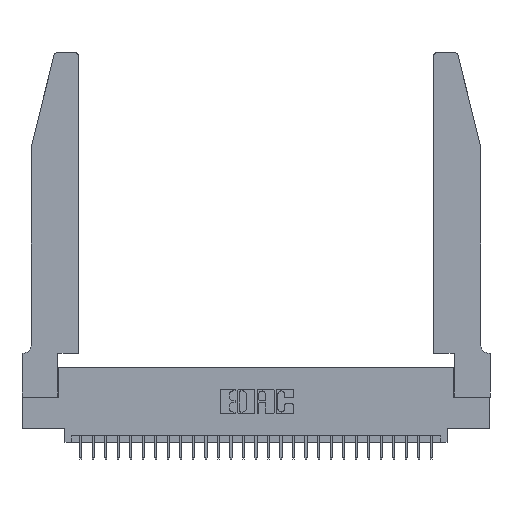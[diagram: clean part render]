
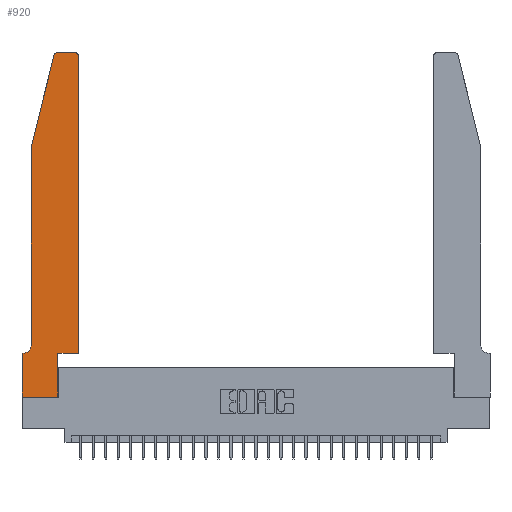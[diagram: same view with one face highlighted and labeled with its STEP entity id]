
A CAD part, top view. The second image highlights one B-rep face of the part: STEP entity #920.
In plain terms, the highlighted planar face has unit normal (0, 0, 1).
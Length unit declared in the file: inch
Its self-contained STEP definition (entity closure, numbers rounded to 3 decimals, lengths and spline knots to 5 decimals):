
#200 = PLANE ( 'NONE',  #16085 ) ;
#347 = LINE ( 'NONE', #27512, #17475 ) ;
#394 = EDGE_CURVE ( 'NONE', #6645, #23849, #20390, .T. ) ;
#507 = FACE_OUTER_BOUND ( 'NONE', #16036, .T. ) ;
#920 = ADVANCED_FACE ( 'NONE', ( #507 ), #200, .T. ) ;
#1801 = CARTESIAN_POINT ( 'NONE',  ( 0.0755, 0.35, 0.37 ) ) ;
#1813 = CARTESIAN_POINT ( 'NONE',  ( 0.0755, 2., 0.37 ) ) ;
#2017 = CARTESIAN_POINT ( 'NONE',  ( 0., 0., 0.37 ) ) ;
#2040 = VERTEX_POINT ( 'NONE', #2017 ) ;
#2989 = DIRECTION ( 'NONE',  ( -1., 0., 0. ) ) ;
#3089 = EDGE_CURVE ( 'NONE', #14643, #23645, #22229, .T. ) ;
#3415 = ORIENTED_EDGE ( 'NONE', *, *, #20732, .T. ) ;
#3640 = VECTOR ( 'NONE', #22770, 39.37008 ) ;
#4037 = CARTESIAN_POINT ( 'NONE',  ( 0.4505, 0.35, 0.37 ) ) ;
#4064 = LINE ( 'NONE', #24223, #6654 ) ;
#4484 = ORIENTED_EDGE ( 'NONE', *, *, #28660, .T. ) ;
#4575 = ORIENTED_EDGE ( 'NONE', *, *, #14215, .T. ) ;
#4797 = CARTESIAN_POINT ( 'NONE',  ( 0.284, 2.75, 0.37 ) ) ;
#5104 = CARTESIAN_POINT ( 'NONE',  ( 0., 0.35, 0.37 ) ) ;
#5279 = EDGE_CURVE ( 'NONE', #23849, #8082, #4064, .T. ) ;
#5374 = CARTESIAN_POINT ( 'NONE',  ( 0.2605, 2.75, 0.37 ) ) ;
#6134 = ORIENTED_EDGE ( 'NONE', *, *, #21720, .T. ) ;
#6453 = DIRECTION ( 'NONE',  ( -0.239, -0.971, 0. ) ) ;
#6645 = VERTEX_POINT ( 'NONE', #4797 ) ;
#6654 = VECTOR ( 'NONE', #6453, 39.37008 ) ;
#6843 = DIRECTION ( 'NONE',  ( 0., 1., 0. ) ) ;
#7436 = VECTOR ( 'NONE', #25301, 39.37008 ) ;
#7520 = DIRECTION ( 'NONE',  ( 0., 0., 1. ) ) ;
#7911 = AXIS2_PLACEMENT_3D ( 'NONE', #22703, #14601, #21188 ) ;
#8021 = VERTEX_POINT ( 'NONE', #9719 ) ;
#8082 = VERTEX_POINT ( 'NONE', #1813 ) ;
#8437 = LINE ( 'NONE', #26649, #12352 ) ;
#8638 = ORIENTED_EDGE ( 'NONE', *, *, #3089, .T. ) ;
#8874 = VECTOR ( 'NONE', #15815, 39.37008 ) ;
#9189 = CARTESIAN_POINT ( 'NONE',  ( 0.4505, 0.35, 0.37 ) ) ;
#9289 = ORIENTED_EDGE ( 'NONE', *, *, #21167, .T. ) ;
#9345 = DIRECTION ( 'NONE',  ( 1., 0., 0. ) ) ;
#9667 = CARTESIAN_POINT ( 'NONE',  ( 0.2865, 0., 0.37 ) ) ;
#9719 = CARTESIAN_POINT ( 'NONE',  ( 0.2865, 0.35, 0.37 ) ) ;
#10353 = VECTOR ( 'NONE', #10896, 39.37008 ) ;
#10664 = VERTEX_POINT ( 'NONE', #26096 ) ;
#10896 = DIRECTION ( 'NONE',  ( -1., 0., 0. ) ) ;
#10957 = VERTEX_POINT ( 'NONE', #18164 ) ;
#11267 = ORIENTED_EDGE ( 'NONE', *, *, #394, .T. ) ;
#11859 = CARTESIAN_POINT ( 'NONE',  ( 0., 0., 0.37 ) ) ;
#12352 = VECTOR ( 'NONE', #17390, 39.37008 ) ;
#14215 = EDGE_CURVE ( 'NONE', #10664, #6645, #25700, .T. ) ;
#14601 = DIRECTION ( 'NONE',  ( 0., 0., -1. ) ) ;
#14643 = VERTEX_POINT ( 'NONE', #21169 ) ;
#15305 = EDGE_CURVE ( 'NONE', #23645, #2040, #20818, .T. ) ;
#15375 = EDGE_CURVE ( 'NONE', #10957, #10664, #24615, .T. ) ;
#15485 = VECTOR ( 'NONE', #2989, 39.37008 ) ;
#15815 = DIRECTION ( 'NONE',  ( 1., 0., 0. ) ) ;
#16036 = EDGE_LOOP ( 'NONE', ( #4575, #11267, #16542, #6134, #18765, #8638, #23302, #3415, #18754, #9289, #4484, #24400 ) ) ;
#16085 = AXIS2_PLACEMENT_3D ( 'NONE', #5104, #18556, #27359 ) ;
#16542 = ORIENTED_EDGE ( 'NONE', *, *, #5279, .T. ) ;
#16635 = VERTEX_POINT ( 'NONE', #24690 ) ;
#17390 = DIRECTION ( 'NONE',  ( 0., 1., 0. ) ) ;
#17475 = VECTOR ( 'NONE', #25126, 39.37008 ) ;
#18074 = CARTESIAN_POINT ( 'NONE',  ( 0., 0., 0.37 ) ) ;
#18164 = CARTESIAN_POINT ( 'NONE',  ( 0.4505, 2.72, 0.37 ) ) ;
#18208 = LINE ( 'NONE', #27311, #21998 ) ;
#18556 = DIRECTION ( 'NONE',  ( 0., 0., 1. ) ) ;
#18601 = EDGE_CURVE ( 'NONE', #16635, #14643, #19356, .T. ) ;
#18725 = CARTESIAN_POINT ( 'NONE',  ( 0.4205, 2.72, 0.37 ) ) ;
#18754 = ORIENTED_EDGE ( 'NONE', *, *, #26317, .T. ) ;
#18765 = ORIENTED_EDGE ( 'NONE', *, *, #18601, .T. ) ;
#18915 = VERTEX_POINT ( 'NONE', #9667 ) ;
#19356 = CIRCLE ( 'NONE', #7911, 0.07 ) ;
#20390 = CIRCLE ( 'NONE', #29455, 0.03 ) ;
#20539 = VERTEX_POINT ( 'NONE', #4037 ) ;
#20732 = EDGE_CURVE ( 'NONE', #2040, #18915, #29428, .T. ) ;
#20818 = LINE ( 'NONE', #11859, #7436 ) ;
#21120 = DIRECTION ( 'NONE',  ( 0., 0., 1. ) ) ;
#21167 = EDGE_CURVE ( 'NONE', #8021, #20539, #25458, .T. ) ;
#21169 = CARTESIAN_POINT ( 'NONE',  ( 0.0055, 0.35, 0.37 ) ) ;
#21188 = DIRECTION ( 'NONE',  ( -1., 0., 0. ) ) ;
#21720 = EDGE_CURVE ( 'NONE', #8082, #16635, #347, .T. ) ;
#21998 = VECTOR ( 'NONE', #6843, 39.37008 ) ;
#22229 = LINE ( 'NONE', #1801, #10353 ) ;
#22693 = AXIS2_PLACEMENT_3D ( 'NONE', #18725, #7520, #27832 ) ;
#22703 = CARTESIAN_POINT ( 'NONE',  ( 0.0055, 0.42, 0.37 ) ) ;
#22770 = DIRECTION ( 'NONE',  ( 1., 0., 0. ) ) ;
#23302 = ORIENTED_EDGE ( 'NONE', *, *, #15305, .T. ) ;
#23645 = VERTEX_POINT ( 'NONE', #26277 ) ;
#23849 = VERTEX_POINT ( 'NONE', #27601 ) ;
#24223 = CARTESIAN_POINT ( 'NONE',  ( 0.0755, 2., 0.37 ) ) ;
#24400 = ORIENTED_EDGE ( 'NONE', *, *, #15375, .T. ) ;
#24615 = CIRCLE ( 'NONE', #22693, 0.03 ) ;
#24690 = CARTESIAN_POINT ( 'NONE',  ( 0.0755, 0.42, 0.37 ) ) ;
#25126 = DIRECTION ( 'NONE',  ( 0., -1., 0. ) ) ;
#25301 = DIRECTION ( 'NONE',  ( 0., -1., 0. ) ) ;
#25458 = LINE ( 'NONE', #9189, #3640 ) ;
#25700 = LINE ( 'NONE', #5374, #15485 ) ;
#26096 = CARTESIAN_POINT ( 'NONE',  ( 0.4205, 2.75, 0.37 ) ) ;
#26277 = CARTESIAN_POINT ( 'NONE',  ( 0., 0.35, 0.37 ) ) ;
#26317 = EDGE_CURVE ( 'NONE', #18915, #8021, #8437, .T. ) ;
#26649 = CARTESIAN_POINT ( 'NONE',  ( 0.2865, 0.35, 0.37 ) ) ;
#27311 = CARTESIAN_POINT ( 'NONE',  ( 0.4505, 0.35, 0.37 ) ) ;
#27359 = DIRECTION ( 'NONE',  ( 1., 0., 0. ) ) ;
#27512 = CARTESIAN_POINT ( 'NONE',  ( 0.0755, 2., 0.37 ) ) ;
#27601 = CARTESIAN_POINT ( 'NONE',  ( 0.25487, 2.72718, 0.37 ) ) ;
#27832 = DIRECTION ( 'NONE',  ( 1., 0., 0. ) ) ;
#28148 = CARTESIAN_POINT ( 'NONE',  ( 0.284, 2.72, 0.37 ) ) ;
#28660 = EDGE_CURVE ( 'NONE', #20539, #10957, #18208, .T. ) ;
#29428 = LINE ( 'NONE', #18074, #8874 ) ;
#29455 = AXIS2_PLACEMENT_3D ( 'NONE', #28148, #21120, #9345 ) ;
